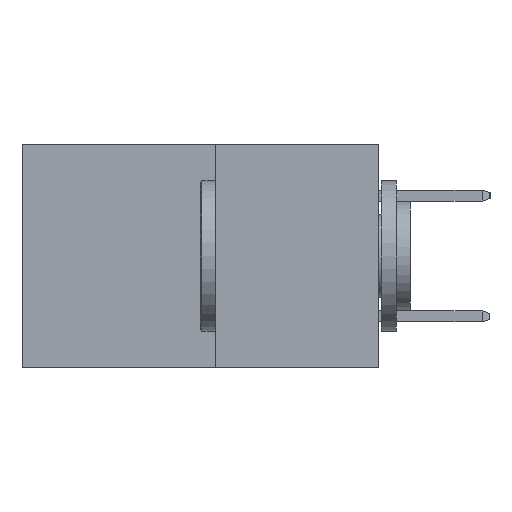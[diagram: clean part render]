
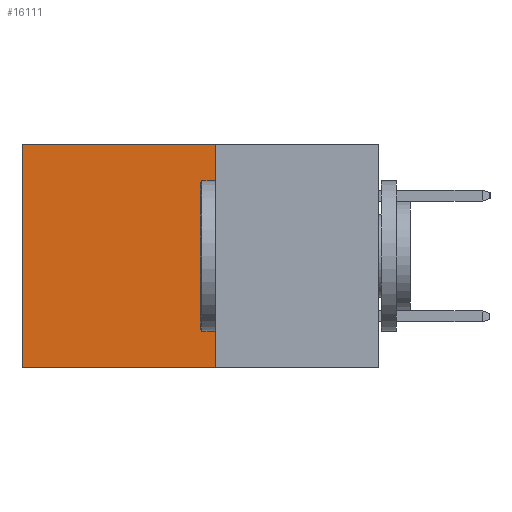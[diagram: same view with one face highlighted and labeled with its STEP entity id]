
A CAD part, left-side view. The second image highlights one B-rep face of the part: STEP entity #16111.
In plain terms, the highlighted planar face has unit normal (-1, 0, 0).
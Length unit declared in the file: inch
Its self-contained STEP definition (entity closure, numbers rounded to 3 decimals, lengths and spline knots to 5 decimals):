
#208 = EDGE_CURVE ( 'NONE', #15478, #2592, #11158, .T. ) ;
#224 = CARTESIAN_POINT ( 'NONE',  ( 0.277, 0.27, -0.37 ) ) ;
#760 = CARTESIAN_POINT ( 'NONE',  ( 0.277, 0.59, -0.37 ) ) ;
#1108 = DIRECTION ( 'NONE',  ( 1., 0., 0. ) ) ;
#1709 = LINE ( 'NONE', #11388, #6267 ) ;
#2197 = ORIENTED_EDGE ( 'NONE', *, *, #9354, .F. ) ;
#2592 = VERTEX_POINT ( 'NONE', #760 ) ;
#4317 = CARTESIAN_POINT ( 'NONE',  ( 0.277, 0.27, 0. ) ) ;
#4907 = PLANE ( 'NONE',  #20140 ) ;
#6081 = DIRECTION ( 'NONE',  ( 0., 1., 0. ) ) ;
#6267 = VECTOR ( 'NONE', #9635, 39.37008 ) ;
#9354 = EDGE_CURVE ( 'NONE', #22637, #13521, #14205, .T. ) ;
#9635 = DIRECTION ( 'NONE',  ( 0., 1., 0. ) ) ;
#10201 = VECTOR ( 'NONE', #6081, 39.37008 ) ;
#10467 = ORIENTED_EDGE ( 'NONE', *, *, #208, .T. ) ;
#10957 = ORIENTED_EDGE ( 'NONE', *, *, #16711, .T. ) ;
#11158 = LINE ( 'NONE', #11590, #20565 ) ;
#11388 = CARTESIAN_POINT ( 'NONE',  ( 0.277, 0.27, 0. ) ) ;
#11590 = CARTESIAN_POINT ( 'NONE',  ( 0.277, 0.59, -0.37 ) ) ;
#12014 = CARTESIAN_POINT ( 'NONE',  ( 0.277, 0.27, -0.37 ) ) ;
#13521 = VERTEX_POINT ( 'NONE', #15254 ) ;
#13607 = VECTOR ( 'NONE', #23270, 39.37008 ) ;
#14205 = LINE ( 'NONE', #12014, #13607 ) ;
#14604 = DIRECTION ( 'NONE',  ( 0., 0., -1. ) ) ;
#15254 = CARTESIAN_POINT ( 'NONE',  ( 0.277, 0.27, -0.37 ) ) ;
#15277 = LINE ( 'NONE', #224, #10201 ) ;
#15478 = VERTEX_POINT ( 'NONE', #16531 ) ;
#16111 = ADVANCED_FACE ( 'NONE', ( #20599 ), #4907, .F. ) ;
#16531 = CARTESIAN_POINT ( 'NONE',  ( 0.277, 0.59, 0. ) ) ;
#16533 = DIRECTION ( 'NONE',  ( 0., 0., -1. ) ) ;
#16711 = EDGE_CURVE ( 'NONE', #22637, #15478, #1709, .T. ) ;
#17068 = EDGE_CURVE ( 'NONE', #13521, #2592, #15277, .T. ) ;
#20140 = AXIS2_PLACEMENT_3D ( 'NONE', #21983, #1108, #14604 ) ;
#20565 = VECTOR ( 'NONE', #16533, 39.37008 ) ;
#20599 = FACE_OUTER_BOUND ( 'NONE', #23278, .T. ) ;
#21983 = CARTESIAN_POINT ( 'NONE',  ( 0.277, 0.27, -0.37 ) ) ;
#22637 = VERTEX_POINT ( 'NONE', #4317 ) ;
#23270 = DIRECTION ( 'NONE',  ( 0., 0., -1. ) ) ;
#23278 = EDGE_LOOP ( 'NONE', ( #10467, #24162, #2197, #10957 ) ) ;
#24162 = ORIENTED_EDGE ( 'NONE', *, *, #17068, .F. ) ;
